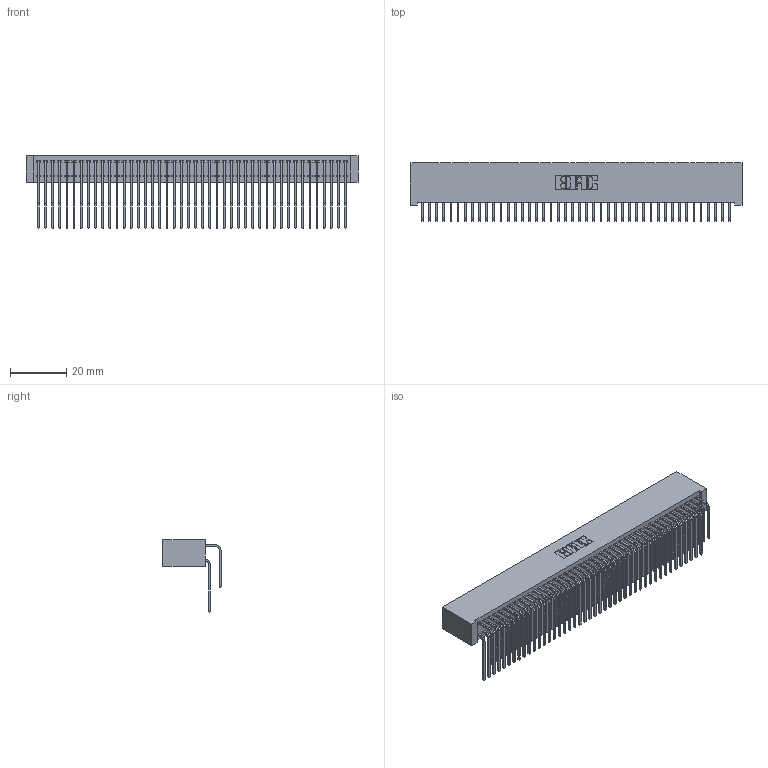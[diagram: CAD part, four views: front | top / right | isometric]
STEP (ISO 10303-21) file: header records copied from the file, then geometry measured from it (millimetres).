
FILE_DESCRIPTION (( 'STEP AP203' ), '1' );
FILE_NAME ('342-088-559-201.STEP', '2018-08-14T00:43:16', ( '' ), ( '' ), 'SwSTEP 2.0', 'SolidWorks 2016', '' );
FILE_SCHEMA (( 'CONFIG_CONTROL_DESIGN' ));
Length unit declared in the file: inch
Products named in the file (4): 342-088-559-201; 342 Part_Lugless; 345-292-001_558 559 Tail - 1; 345-292-001_559 Tail - 2
Assembly tree (89 placements, depth 2):
  342-088-559-201
    342 Part_Lugless
    345-292-001_558 559 Tail - 1  x44
    345-292-001_559 Tail - 2  x44
Bounding box: 118.01 x 20.64 x 25.78 mm (x, y, z)
Volume: 11559.7 mm3; surface area: 21608.2 mm2
Topology: 89 solids, 89 shells, 4854 faces, 14443 edges, 9510 vertices
Faces by surface type: plane 3406, cylinder 1448
Entity records: 29423 total; most frequent: CARTESIAN_POINT 4921, ORIENTED_EDGE 4806, DIRECTION 4175, EDGE_CURVE 2403, VECTOR 2243, LINE 2243, VERTEX_POINT 1598, AXIS2_PLACEMENT_3D 966
